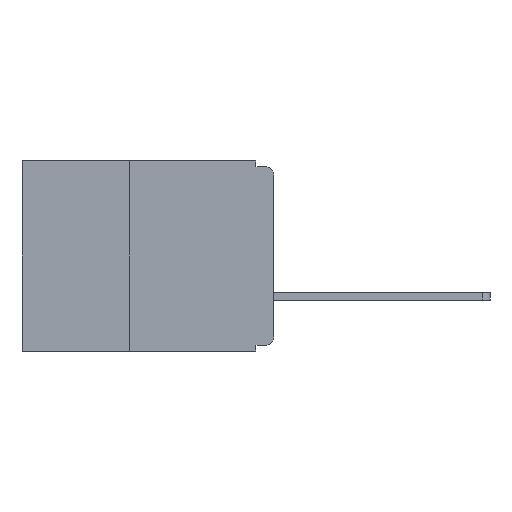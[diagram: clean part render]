
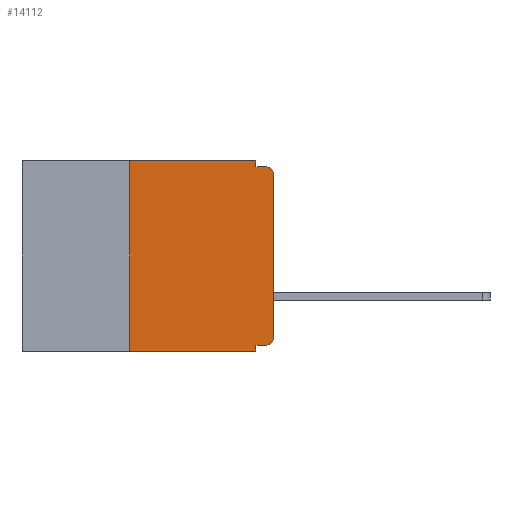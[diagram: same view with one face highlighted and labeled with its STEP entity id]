
A CAD part, left-side view. The second image highlights one B-rep face of the part: STEP entity #14112.
In plain terms, the highlighted planar face has unit normal (-1, 0, 0).
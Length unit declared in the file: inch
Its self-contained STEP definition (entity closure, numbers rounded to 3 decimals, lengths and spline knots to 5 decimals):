
#707 = ORIENTED_EDGE ( 'NONE', *, *, #4589, .F. ) ;
#733 = DIRECTION ( 'NONE',  ( 0., 0., 1. ) ) ;
#1131 = DIRECTION ( 'NONE',  ( -1., 0., 0. ) ) ;
#1344 = CARTESIAN_POINT ( 'NONE',  ( 0., 0.437, -0.33 ) ) ;
#1375 = AXIS2_PLACEMENT_3D ( 'NONE', #7807, #16127, #12113 ) ;
#1386 = CARTESIAN_POINT ( 'NONE',  ( 0., 0.031, 0. ) ) ;
#1629 = FACE_OUTER_BOUND ( 'NONE', #16663, .T. ) ;
#2751 = EDGE_CURVE ( 'NONE', #25213, #27248, #26705, .T. ) ;
#2923 = ORIENTED_EDGE ( 'NONE', *, *, #25551, .F. ) ;
#3465 = CARTESIAN_POINT ( 'NONE',  ( 0., 0.031, -0.01 ) ) ;
#4589 = EDGE_CURVE ( 'NONE', #14187, #26537, #6872, .T. ) ;
#4956 = DIRECTION ( 'NONE',  ( 0., 0., -1. ) ) ;
#5152 = VERTEX_POINT ( 'NONE', #15352 ) ;
#5242 = VECTOR ( 'NONE', #22545, 39.37008 ) ;
#5455 = LINE ( 'NONE', #7128, #16066 ) ;
#5615 = VERTEX_POINT ( 'NONE', #17154 ) ;
#6274 = DIRECTION ( 'NONE',  ( 0., 1., 0. ) ) ;
#6486 = ORIENTED_EDGE ( 'NONE', *, *, #2751, .T. ) ;
#6589 = VERTEX_POINT ( 'NONE', #3465 ) ;
#6872 = LINE ( 'NONE', #20044, #7518 ) ;
#6886 = AXIS2_PLACEMENT_3D ( 'NONE', #12776, #27418, #14868 ) ;
#7128 = CARTESIAN_POINT ( 'NONE',  ( 0., 0.031, -0.33 ) ) ;
#7184 = EDGE_CURVE ( 'NONE', #5152, #8245, #17305, .T. ) ;
#7398 = AXIS2_PLACEMENT_3D ( 'NONE', #14149, #1131, #16258 ) ;
#7455 = EDGE_CURVE ( 'NONE', #5615, #24203, #27454, .T. ) ;
#7518 = VECTOR ( 'NONE', #9601, 39.37008 ) ;
#7807 = CARTESIAN_POINT ( 'NONE',  ( 0., 0.437, 0. ) ) ;
#8245 = VERTEX_POINT ( 'NONE', #9032 ) ;
#8962 = VECTOR ( 'NONE', #24836, 39.37008 ) ;
#9032 = CARTESIAN_POINT ( 'NONE',  ( 0., 0., -0.305 ) ) ;
#9284 = LINE ( 'NONE', #11692, #14217 ) ;
#9601 = DIRECTION ( 'NONE',  ( 0., -1., 0. ) ) ;
#9616 = ORIENTED_EDGE ( 'NONE', *, *, #7184, .T. ) ;
#9651 = LINE ( 'NONE', #1386, #8962 ) ;
#9886 = ORIENTED_EDGE ( 'NONE', *, *, #7455, .T. ) ;
#9996 = PLANE ( 'NONE',  #1375 ) ;
#10527 = CARTESIAN_POINT ( 'NONE',  ( 0., 0.031, -0.32 ) ) ;
#10957 = LINE ( 'NONE', #12142, #5242 ) ;
#11664 = ORIENTED_EDGE ( 'NONE', *, *, #22489, .F. ) ;
#11692 = CARTESIAN_POINT ( 'NONE',  ( 0., 0., 0. ) ) ;
#11718 = ORIENTED_EDGE ( 'NONE', *, *, #17973, .F. ) ;
#12113 = DIRECTION ( 'NONE',  ( 0., 0., -1. ) ) ;
#12142 = CARTESIAN_POINT ( 'NONE',  ( 0., 0., -0.01 ) ) ;
#12776 = CARTESIAN_POINT ( 'NONE',  ( 0., 0.015, -0.025 ) ) ;
#12968 = ORIENTED_EDGE ( 'NONE', *, *, #21233, .F. ) ;
#13362 = EDGE_CURVE ( 'NONE', #8245, #5615, #9284, .T. ) ;
#13502 = EDGE_CURVE ( 'NONE', #6589, #24203, #10957, .T. ) ;
#13649 = VECTOR ( 'NONE', #18699, 39.37008 ) ;
#14112 = ADVANCED_FACE ( 'NONE', ( #1629 ), #9996, .F. ) ;
#14121 = CARTESIAN_POINT ( 'NONE',  ( 0., 0.015, -0.01 ) ) ;
#14149 = CARTESIAN_POINT ( 'NONE',  ( 0., 0.015, -0.305 ) ) ;
#14187 = VERTEX_POINT ( 'NONE', #18594 ) ;
#14217 = VECTOR ( 'NONE', #733, 39.37008 ) ;
#14868 = DIRECTION ( 'NONE',  ( 0., 0., -1. ) ) ;
#14951 = LINE ( 'NONE', #24929, #13649 ) ;
#15352 = CARTESIAN_POINT ( 'NONE',  ( 0., 0.015, -0.32 ) ) ;
#15944 = CARTESIAN_POINT ( 'NONE',  ( 0., 0.031, 0. ) ) ;
#16066 = VECTOR ( 'NONE', #4956, 39.37008 ) ;
#16127 = DIRECTION ( 'NONE',  ( 1., 0., 0. ) ) ;
#16258 = DIRECTION ( 'NONE',  ( 0., 0., -1. ) ) ;
#16663 = EDGE_LOOP ( 'NONE', ( #24307, #9886, #26958, #11664, #707, #11718, #6486, #12968, #2923, #9616 ) ) ;
#16672 = VECTOR ( 'NONE', #6274, 39.37008 ) ;
#17154 = CARTESIAN_POINT ( 'NONE',  ( 0., 0., -0.025 ) ) ;
#17305 = CIRCLE ( 'NONE', #7398, 0.015 ) ;
#17331 = LINE ( 'NONE', #20986, #16672 ) ;
#17743 = CARTESIAN_POINT ( 'NONE',  ( 0., 0.25, -0.33 ) ) ;
#17973 = EDGE_CURVE ( 'NONE', #25213, #14187, #14951, .T. ) ;
#18594 = CARTESIAN_POINT ( 'NONE',  ( 0., 0.25, 0. ) ) ;
#18699 = DIRECTION ( 'NONE',  ( 0., 0., 1. ) ) ;
#20044 = CARTESIAN_POINT ( 'NONE',  ( 0., 0.437, 0. ) ) ;
#20228 = CARTESIAN_POINT ( 'NONE',  ( 0., 0.031, -0.33 ) ) ;
#20467 = VECTOR ( 'NONE', #26896, 39.37008 ) ;
#20986 = CARTESIAN_POINT ( 'NONE',  ( 0., 0., -0.32 ) ) ;
#21017 = VERTEX_POINT ( 'NONE', #10527 ) ;
#21233 = EDGE_CURVE ( 'NONE', #21017, #27248, #5455, .T. ) ;
#22489 = EDGE_CURVE ( 'NONE', #26537, #6589, #9651, .T. ) ;
#22545 = DIRECTION ( 'NONE',  ( 0., -1., 0. ) ) ;
#24203 = VERTEX_POINT ( 'NONE', #14121 ) ;
#24307 = ORIENTED_EDGE ( 'NONE', *, *, #13362, .T. ) ;
#24836 = DIRECTION ( 'NONE',  ( 0., 0., -1. ) ) ;
#24929 = CARTESIAN_POINT ( 'NONE',  ( 0., 0.25, -0.33 ) ) ;
#25213 = VERTEX_POINT ( 'NONE', #17743 ) ;
#25551 = EDGE_CURVE ( 'NONE', #5152, #21017, #17331, .T. ) ;
#26537 = VERTEX_POINT ( 'NONE', #15944 ) ;
#26705 = LINE ( 'NONE', #1344, #20467 ) ;
#26896 = DIRECTION ( 'NONE',  ( 0., -1., 0. ) ) ;
#26958 = ORIENTED_EDGE ( 'NONE', *, *, #13502, .F. ) ;
#27248 = VERTEX_POINT ( 'NONE', #20228 ) ;
#27418 = DIRECTION ( 'NONE',  ( -1., 0., 0. ) ) ;
#27454 = CIRCLE ( 'NONE', #6886, 0.015 ) ;
